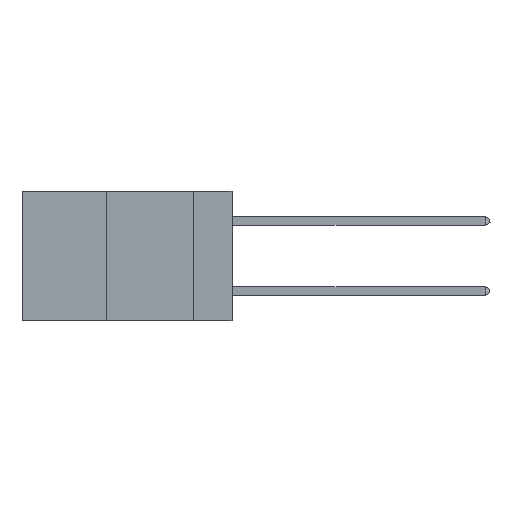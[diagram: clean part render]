
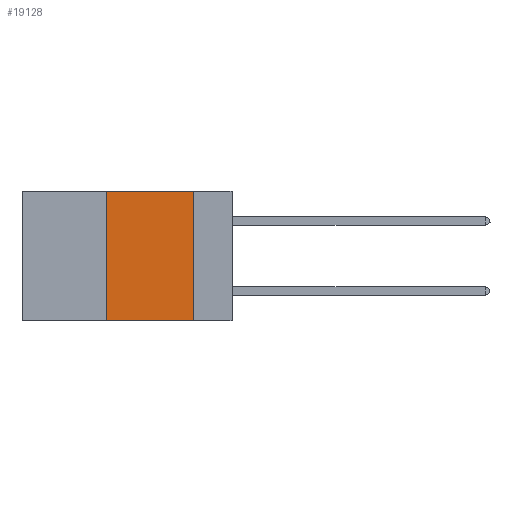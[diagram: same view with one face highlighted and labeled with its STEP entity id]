
A CAD part, left-side view. The second image highlights one B-rep face of the part: STEP entity #19128.
In plain terms, the highlighted planar face has unit normal (-1, 0, 0).
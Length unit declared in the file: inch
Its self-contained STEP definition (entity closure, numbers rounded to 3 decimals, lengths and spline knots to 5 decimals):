
#446 = LINE ( 'NONE', #16547, #16926 ) ;
#814 = ORIENTED_EDGE ( 'NONE', *, *, #12413, .F. ) ;
#911 = DIRECTION ( 'NONE',  ( 0., -1., 0. ) ) ;
#1367 = ORIENTED_EDGE ( 'NONE', *, *, #8995, .T. ) ;
#2128 = VERTEX_POINT ( 'NONE', #12779 ) ;
#2210 = VECTOR ( 'NONE', #911, 39.37008 ) ;
#3051 = EDGE_CURVE ( 'NONE', #8271, #2128, #20313, .T. ) ;
#5632 = DIRECTION ( 'NONE',  ( 0., 0., -1. ) ) ;
#6064 = CARTESIAN_POINT ( 'NONE',  ( 0., 0.6, 0. ) ) ;
#7134 = DIRECTION ( 'NONE',  ( 0., 0., 1. ) ) ;
#7613 = EDGE_LOOP ( 'NONE', ( #8571, #814, #9561, #1367 ) ) ;
#7693 = DIRECTION ( 'NONE',  ( 1., 0., 0. ) ) ;
#8271 = VERTEX_POINT ( 'NONE', #8930 ) ;
#8300 = VERTEX_POINT ( 'NONE', #16729 ) ;
#8318 = FACE_OUTER_BOUND ( 'NONE', #7613, .T. ) ;
#8571 = ORIENTED_EDGE ( 'NONE', *, *, #15258, .F. ) ;
#8930 = CARTESIAN_POINT ( 'NONE',  ( 0., 0.36, -0.37 ) ) ;
#8995 = EDGE_CURVE ( 'NONE', #8271, #8300, #18446, .T. ) ;
#9338 = LINE ( 'NONE', #11004, #17022 ) ;
#9561 = ORIENTED_EDGE ( 'NONE', *, *, #3051, .F. ) ;
#10669 = CARTESIAN_POINT ( 'NONE',  ( 0., 0.6, -0.37 ) ) ;
#11004 = CARTESIAN_POINT ( 'NONE',  ( 0., 0.6, 0. ) ) ;
#12314 = VECTOR ( 'NONE', #7134, 39.37008 ) ;
#12413 = EDGE_CURVE ( 'NONE', #2128, #14415, #9338, .T. ) ;
#12596 = DIRECTION ( 'NONE',  ( 0., -1., 0. ) ) ;
#12779 = CARTESIAN_POINT ( 'NONE',  ( 0., 0.36, 0. ) ) ;
#14415 = VERTEX_POINT ( 'NONE', #19046 ) ;
#14655 = AXIS2_PLACEMENT_3D ( 'NONE', #6064, #7693, #18429 ) ;
#15258 = EDGE_CURVE ( 'NONE', #14415, #8300, #446, .T. ) ;
#16547 = CARTESIAN_POINT ( 'NONE',  ( 0., 0.11, 0. ) ) ;
#16729 = CARTESIAN_POINT ( 'NONE',  ( 0., 0.11, -0.37 ) ) ;
#16926 = VECTOR ( 'NONE', #5632, 39.37008 ) ;
#17022 = VECTOR ( 'NONE', #12596, 39.37008 ) ;
#17911 = CARTESIAN_POINT ( 'NONE',  ( 0., 0.36, 0. ) ) ;
#18365 = PLANE ( 'NONE',  #14655 ) ;
#18429 = DIRECTION ( 'NONE',  ( 0., 0., -1. ) ) ;
#18446 = LINE ( 'NONE', #10669, #2210 ) ;
#19046 = CARTESIAN_POINT ( 'NONE',  ( 0., 0.11, 0. ) ) ;
#19128 = ADVANCED_FACE ( 'NONE', ( #8318 ), #18365, .F. ) ;
#20313 = LINE ( 'NONE', #17911, #12314 ) ;
